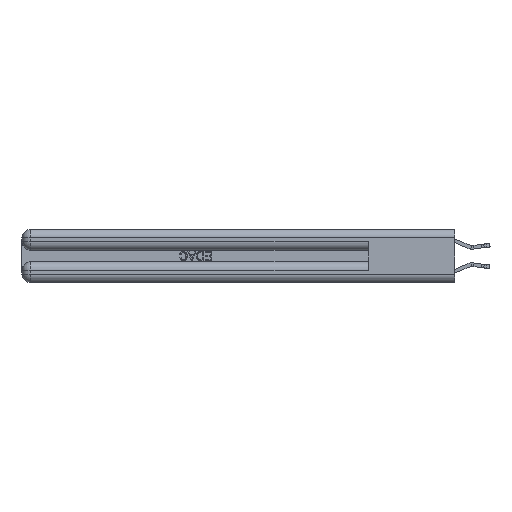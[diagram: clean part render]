
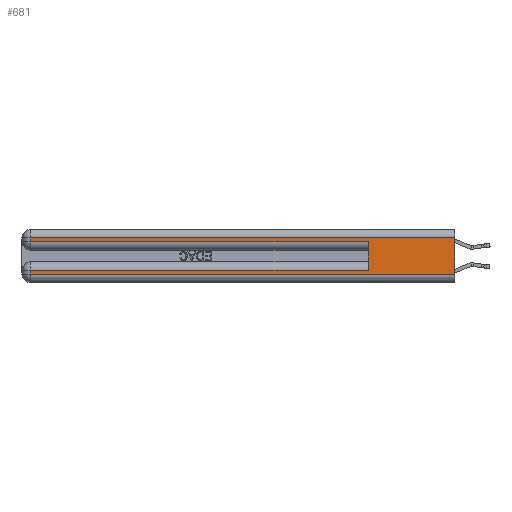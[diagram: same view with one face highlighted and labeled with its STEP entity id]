
A CAD part, left-side view. The second image highlights one B-rep face of the part: STEP entity #681.
In plain terms, the highlighted planar face has unit normal (-1, 0, 0).
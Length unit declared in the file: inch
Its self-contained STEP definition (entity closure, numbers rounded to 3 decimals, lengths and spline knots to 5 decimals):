
#5 = CARTESIAN_POINT ( 'NONE',  ( 0., 0.6, 0.285 ) ) ;
#291 = EDGE_CURVE ( 'NONE', #23556, #4849, #14006, .T. ) ;
#313 = VERTEX_POINT ( 'NONE', #27796 ) ;
#552 = DIRECTION ( 'NONE',  ( 0., 0., -1. ) ) ;
#681 = ADVANCED_FACE ( 'NONE', ( #34544 ), #26649, .F. ) ;
#915 = EDGE_CURVE ( 'NONE', #5695, #1698, #7905, .T. ) ;
#1081 = CARTESIAN_POINT ( 'NONE',  ( 0., 0.6, 0.085 ) ) ;
#1698 = VERTEX_POINT ( 'NONE', #5 ) ;
#1799 = CARTESIAN_POINT ( 'NONE',  ( 0., 0.6, 0.145 ) ) ;
#2540 = CARTESIAN_POINT ( 'NONE',  ( 0., 0., 0.37 ) ) ;
#3335 = DIRECTION ( 'NONE',  ( 0., 1., 0. ) ) ;
#4849 = VERTEX_POINT ( 'NONE', #6095 ) ;
#5280 = CARTESIAN_POINT ( 'NONE',  ( 0., 0., 0.285 ) ) ;
#5404 = VERTEX_POINT ( 'NONE', #20454 ) ;
#5695 = VERTEX_POINT ( 'NONE', #1081 ) ;
#6095 = CARTESIAN_POINT ( 'NONE',  ( 0., 2.94, 0.285 ) ) ;
#6135 = CARTESIAN_POINT ( 'NONE',  ( 0., 0., 0.06 ) ) ;
#7191 = ORIENTED_EDGE ( 'NONE', *, *, #915, .F. ) ;
#7724 = VECTOR ( 'NONE', #552, 39.37008 ) ;
#7730 = LINE ( 'NONE', #6135, #34752 ) ;
#7905 = LINE ( 'NONE', #1799, #25508 ) ;
#8293 = DIRECTION ( 'NONE',  ( 0., 0., -1. ) ) ;
#8983 = LINE ( 'NONE', #10194, #23082 ) ;
#10194 = CARTESIAN_POINT ( 'NONE',  ( 0., 0., 0.31 ) ) ;
#10750 = LINE ( 'NONE', #2540, #19371 ) ;
#11142 = CARTESIAN_POINT ( 'NONE',  ( 0., 0., 0.37 ) ) ;
#11254 = EDGE_CURVE ( 'NONE', #4849, #1698, #27981, .T. ) ;
#11697 = EDGE_CURVE ( 'NONE', #5404, #313, #10750, .T. ) ;
#11820 = EDGE_CURVE ( 'NONE', #21429, #15651, #33524, .T. ) ;
#13337 = DIRECTION ( 'NONE',  ( 1., 0., 0. ) ) ;
#13617 = DIRECTION ( 'NONE',  ( 0., -1., 0. ) ) ;
#14006 = LINE ( 'NONE', #34560, #32403 ) ;
#14495 = ORIENTED_EDGE ( 'NONE', *, *, #11254, .T. ) ;
#14884 = VECTOR ( 'NONE', #3335, 39.37008 ) ;
#14918 = CARTESIAN_POINT ( 'NONE',  ( 0., 2.94, 0.06 ) ) ;
#15527 = ORIENTED_EDGE ( 'NONE', *, *, #31799, .T. ) ;
#15651 = VERTEX_POINT ( 'NONE', #14918 ) ;
#16000 = DIRECTION ( 'NONE',  ( 0., 1., 0. ) ) ;
#16989 = AXIS2_PLACEMENT_3D ( 'NONE', #11142, #13337, #8293 ) ;
#19371 = VECTOR ( 'NONE', #30005, 39.37008 ) ;
#19724 = EDGE_LOOP ( 'NONE', ( #27923, #33404, #29605, #14495, #7191, #32686, #34256, #15527 ) ) ;
#19933 = EDGE_CURVE ( 'NONE', #5404, #23556, #8983, .T. ) ;
#20454 = CARTESIAN_POINT ( 'NONE',  ( 0., 0., 0.31 ) ) ;
#20650 = VECTOR ( 'NONE', #13617, 39.37008 ) ;
#20701 = DIRECTION ( 'NONE',  ( 0., 0., -1. ) ) ;
#21429 = VERTEX_POINT ( 'NONE', #25427 ) ;
#23082 = VECTOR ( 'NONE', #16000, 39.37008 ) ;
#23556 = VERTEX_POINT ( 'NONE', #26695 ) ;
#25256 = EDGE_CURVE ( 'NONE', #5695, #21429, #26469, .T. ) ;
#25409 = CARTESIAN_POINT ( 'NONE',  ( 0., 0., 0.085 ) ) ;
#25427 = CARTESIAN_POINT ( 'NONE',  ( 0., 2.94, 0.085 ) ) ;
#25508 = VECTOR ( 'NONE', #26427, 39.37008 ) ;
#26427 = DIRECTION ( 'NONE',  ( 0., 0., 1. ) ) ;
#26469 = LINE ( 'NONE', #25409, #14884 ) ;
#26649 = PLANE ( 'NONE',  #16989 ) ;
#26695 = CARTESIAN_POINT ( 'NONE',  ( 0., 2.94, 0.31 ) ) ;
#27796 = CARTESIAN_POINT ( 'NONE',  ( 0., 0., 0.06 ) ) ;
#27923 = ORIENTED_EDGE ( 'NONE', *, *, #11697, .F. ) ;
#27981 = LINE ( 'NONE', #5280, #20650 ) ;
#28133 = DIRECTION ( 'NONE',  ( 0., -1., 0. ) ) ;
#29605 = ORIENTED_EDGE ( 'NONE', *, *, #291, .T. ) ;
#30005 = DIRECTION ( 'NONE',  ( 0., 0., -1. ) ) ;
#31799 = EDGE_CURVE ( 'NONE', #15651, #313, #7730, .T. ) ;
#32403 = VECTOR ( 'NONE', #20701, 39.37008 ) ;
#32686 = ORIENTED_EDGE ( 'NONE', *, *, #25256, .T. ) ;
#33404 = ORIENTED_EDGE ( 'NONE', *, *, #19933, .T. ) ;
#33524 = LINE ( 'NONE', #33687, #7724 ) ;
#33687 = CARTESIAN_POINT ( 'NONE',  ( 0., 2.94, 0.37 ) ) ;
#34256 = ORIENTED_EDGE ( 'NONE', *, *, #11820, .T. ) ;
#34544 = FACE_OUTER_BOUND ( 'NONE', #19724, .T. ) ;
#34560 = CARTESIAN_POINT ( 'NONE',  ( 0., 2.94, 0.37 ) ) ;
#34752 = VECTOR ( 'NONE', #28133, 39.37008 ) ;
